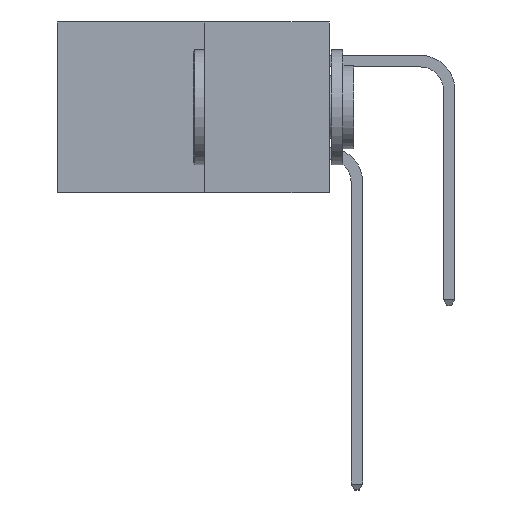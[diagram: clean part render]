
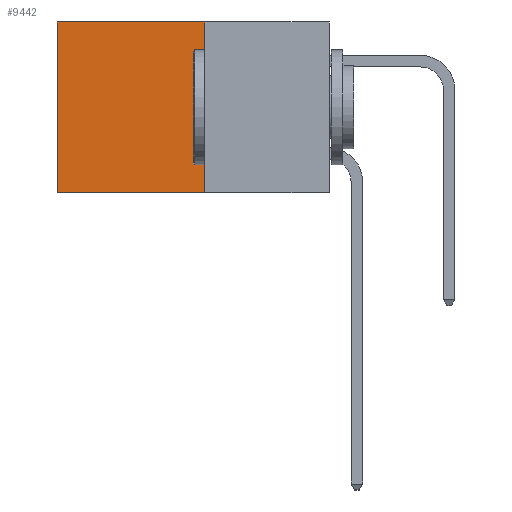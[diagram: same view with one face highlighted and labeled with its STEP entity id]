
A CAD part, left-side view. The second image highlights one B-rep face of the part: STEP entity #9442.
In plain terms, the highlighted planar face has unit normal (-1, 0, 0).
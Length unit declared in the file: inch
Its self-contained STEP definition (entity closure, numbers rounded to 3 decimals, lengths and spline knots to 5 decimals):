
#197 = EDGE_LOOP ( 'NONE', ( #8094, #10513, #294, #8541 ) ) ;
#294 = ORIENTED_EDGE ( 'NONE', *, *, #461, .F. ) ;
#461 = EDGE_CURVE ( 'NONE', #4252, #2366, #9570, .T. ) ;
#1520 = CARTESIAN_POINT ( 'NONE',  ( 0.277, 0.59, -0.37 ) ) ;
#1574 = VECTOR ( 'NONE', #7206, 39.37008 ) ;
#1613 = EDGE_CURVE ( 'NONE', #4252, #4670, #9119, .T. ) ;
#1641 = CARTESIAN_POINT ( 'NONE',  ( 0.277, 0.27, -0.37 ) ) ;
#1942 = LINE ( 'NONE', #8555, #3799 ) ;
#2116 = CARTESIAN_POINT ( 'NONE',  ( 0.277, 0.27, 0. ) ) ;
#2164 = PLANE ( 'NONE',  #11723 ) ;
#2366 = VERTEX_POINT ( 'NONE', #1641 ) ;
#2367 = DIRECTION ( 'NONE',  ( 0., 1., 0. ) ) ;
#3144 = FACE_OUTER_BOUND ( 'NONE', #197, .T. ) ;
#3498 = CARTESIAN_POINT ( 'NONE',  ( 0.277, 0.27, -0.37 ) ) ;
#3799 = VECTOR ( 'NONE', #11225, 39.37008 ) ;
#3942 = EDGE_CURVE ( 'NONE', #2366, #6060, #11277, .T. ) ;
#4007 = CARTESIAN_POINT ( 'NONE',  ( 0.277, 0.27, -0.37 ) ) ;
#4252 = VERTEX_POINT ( 'NONE', #9605 ) ;
#4544 = VECTOR ( 'NONE', #2367, 39.37008 ) ;
#4670 = VERTEX_POINT ( 'NONE', #4875 ) ;
#4875 = CARTESIAN_POINT ( 'NONE',  ( 0.277, 0.59, 0. ) ) ;
#4914 = DIRECTION ( 'NONE',  ( 0., 0., -1. ) ) ;
#6060 = VERTEX_POINT ( 'NONE', #1520 ) ;
#7109 = CARTESIAN_POINT ( 'NONE',  ( 0.277, 0.27, -0.37 ) ) ;
#7206 = DIRECTION ( 'NONE',  ( 0., 1., 0. ) ) ;
#8094 = ORIENTED_EDGE ( 'NONE', *, *, #8099, .T. ) ;
#8099 = EDGE_CURVE ( 'NONE', #4670, #6060, #1942, .T. ) ;
#8541 = ORIENTED_EDGE ( 'NONE', *, *, #1613, .T. ) ;
#8555 = CARTESIAN_POINT ( 'NONE',  ( 0.277, 0.59, -0.37 ) ) ;
#9119 = LINE ( 'NONE', #2116, #4544 ) ;
#9442 = ADVANCED_FACE ( 'NONE', ( #3144 ), #2164, .F. ) ;
#9494 = DIRECTION ( 'NONE',  ( 0., 0., -1. ) ) ;
#9570 = LINE ( 'NONE', #3498, #11385 ) ;
#9605 = CARTESIAN_POINT ( 'NONE',  ( 0.277, 0.27, 0. ) ) ;
#10389 = DIRECTION ( 'NONE',  ( 1., 0., 0. ) ) ;
#10513 = ORIENTED_EDGE ( 'NONE', *, *, #3942, .F. ) ;
#11225 = DIRECTION ( 'NONE',  ( 0., 0., -1. ) ) ;
#11277 = LINE ( 'NONE', #7109, #1574 ) ;
#11385 = VECTOR ( 'NONE', #9494, 39.37008 ) ;
#11723 = AXIS2_PLACEMENT_3D ( 'NONE', #4007, #10389, #4914 ) ;
